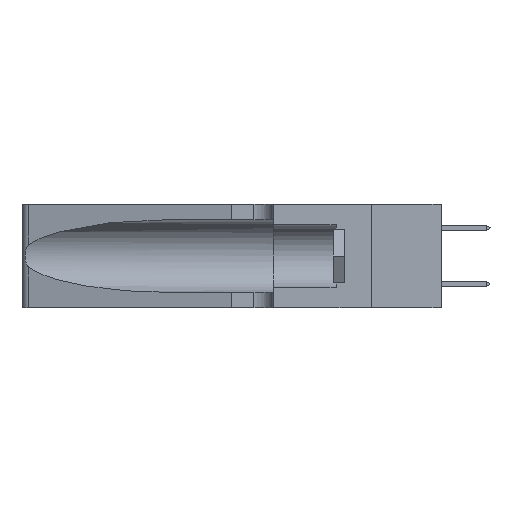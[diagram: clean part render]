
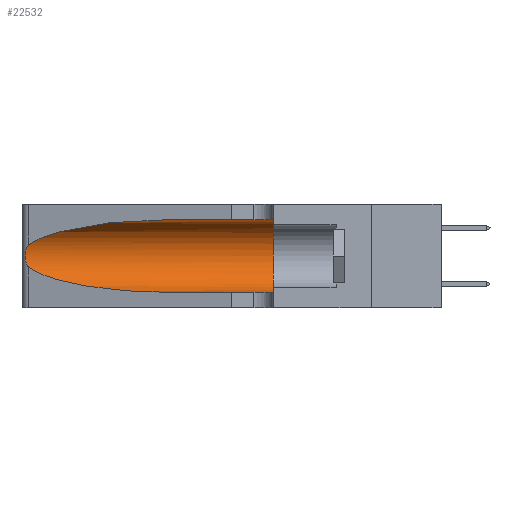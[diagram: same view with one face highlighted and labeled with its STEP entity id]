
A CAD part, left-side view. The second image highlights one B-rep face of the part: STEP entity #22532.
In plain terms, the highlighted cylindrical face has radius 3.308 mm (diameter 6.617 mm), a partial arc.
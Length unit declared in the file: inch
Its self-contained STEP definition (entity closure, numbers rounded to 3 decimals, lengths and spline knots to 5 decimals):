
#297 = CARTESIAN_POINT ( 'NONE',  ( 0.25555, 1.22994, 0.2215 ) ) ;
#299 = VERTEX_POINT ( 'NONE', #20608 ) ;
#329 = VERTEX_POINT ( 'NONE', #12096 ) ;
#825 = CARTESIAN_POINT ( 'NONE',  ( 0.1305, 0.72297, 0.05475 ) ) ;
#1080 = EDGE_CURVE ( 'NONE', #34458, #299, #30667, .T. ) ;
#1246 = LINE ( 'NONE', #26281, #29899 ) ;
#1765 = DIRECTION ( 'NONE',  ( 0., -1., 0. ) ) ;
#2811 = CARTESIAN_POINT ( 'NONE',  ( 0.1305, 0.35, 0.185 ) ) ;
#3085 = CARTESIAN_POINT ( 'NONE',  ( 0.25787, 1.23484, 0.2124 ) ) ;
#3352 = VERTEX_POINT ( 'NONE', #10244 ) ;
#4027 = CYLINDRICAL_SURFACE ( 'NONE', #6193, 0.13025 ) ;
#5576 = DIRECTION ( 'NONE',  ( 0., 0., 1. ) ) ;
#5841 = CARTESIAN_POINT ( 'NONE',  ( 0.26018, 1.23835, 0.19895 ) ) ;
#6193 = AXIS2_PLACEMENT_3D ( 'NONE', #21155, #1765, #29181 ) ;
#7646 = DIRECTION ( 'NONE',  ( 0., -1., 0. ) ) ;
#7833 = AXIS2_PLACEMENT_3D ( 'NONE', #2811, #22202, #5576 ) ;
#8213 = ORIENTED_EDGE ( 'NONE', *, *, #17976, .T. ) ;
#8589 = CARTESIAN_POINT ( 'NONE',  ( 0.26075, 1.23896, 0.178 ) ) ;
#9056 = ORIENTED_EDGE ( 'NONE', *, *, #18629, .T. ) ;
#9939 = CARTESIAN_POINT ( 'NONE',  ( 0.25487, 1.22718, 0.22369 ) ) ;
#10244 = CARTESIAN_POINT ( 'NONE',  ( 0.1305, 0.35, 0.31525 ) ) ;
#11088 = ORIENTED_EDGE ( 'NONE', *, *, #26607, .F. ) ;
#11349 = CARTESIAN_POINT ( 'NONE',  ( 0.25856, 1.23593, 0.16098 ) ) ;
#12096 = CARTESIAN_POINT ( 'NONE',  ( 0.1305, 0.72297, 0.05475 ) ) ;
#12185 = FACE_OUTER_BOUND ( 'NONE', #28134, .T. ) ;
#12963 = ORIENTED_EDGE ( 'NONE', *, *, #1080, .T. ) ;
#14169 = CARTESIAN_POINT ( 'NONE',  ( 0.25639, 1.23186, 0.15144 ) ) ;
#15029 =( BOUNDED_CURVE ( )  B_SPLINE_CURVE ( 3, ( #25590, #31284, #17411, #825 ),
 .UNSPECIFIED., .F., .T. ) 
 B_SPLINE_CURVE_WITH_KNOTS ( ( 4, 4 ),
 ( 3.44316, 4.71239 ),
 .UNSPECIFIED. ) 
 CURVE ( )  GEOMETRIC_REPRESENTATION_ITEM ( )  RATIONAL_B_SPLINE_CURVE ( ( 1., 0.87, 0.87, 1. ) ) 
 REPRESENTATION_ITEM ( '' )  );
#15434 = CARTESIAN_POINT ( 'NONE',  ( 0.1305, 0.72297, 0.31525 ) ) ;
#16083 = EDGE_CURVE ( 'NONE', #19854, #3352, #24612, .T. ) ;
#16888 = CARTESIAN_POINT ( 'NONE',  ( 0.25487, 1.22718, 0.22369 ) ) ;
#17006 = CARTESIAN_POINT ( 'NONE',  ( 0.25487, 1.22718, 0.14631 ) ) ;
#17411 = CARTESIAN_POINT ( 'NONE',  ( 0.18966, 0.96281, 0.05475 ) ) ;
#17976 = EDGE_CURVE ( 'NONE', #299, #329, #15029, .T. ) ;
#18524 = ORIENTED_EDGE ( 'NONE', *, *, #16083, .F. ) ;
#18629 = EDGE_CURVE ( 'NONE', #329, #26020, #1246, .T. ) ;
#19659 = CARTESIAN_POINT ( 'NONE',  ( 0.25639, 1.23184, 0.21858 ) ) ;
#19694 = CARTESIAN_POINT ( 'NONE',  ( 0.1305, 0.72297, 0.31525 ) ) ;
#19854 = VERTEX_POINT ( 'NONE', #19694 ) ;
#20608 = CARTESIAN_POINT ( 'NONE',  ( 0.25487, 1.22718, 0.14631 ) ) ;
#21155 = CARTESIAN_POINT ( 'NONE',  ( 0.1305, 1.61858, 0.185 ) ) ;
#22202 = DIRECTION ( 'NONE',  ( 0., 1., 0. ) ) ;
#22483 = CARTESIAN_POINT ( 'NONE',  ( 0.25854, 1.2359, 0.20912 ) ) ;
#22532 = ADVANCED_FACE ( 'NONE', ( #12185 ), #4027, .F. ) ;
#23453 = ORIENTED_EDGE ( 'NONE', *, *, #35080, .T. ) ;
#23739 = VECTOR ( 'NONE', #7646, 39.37008 ) ;
#24612 = LINE ( 'NONE', #27152, #23739 ) ;
#24699 = CARTESIAN_POINT ( 'NONE',  ( 0.25487, 1.22718, 0.22369 ) ) ;
#24942 = CIRCLE ( 'NONE', #7833, 0.13025 ) ;
#25282 = CARTESIAN_POINT ( 'NONE',  ( 0.26075, 1.23896, 0.19203 ) ) ;
#25590 = CARTESIAN_POINT ( 'NONE',  ( 0.25487, 1.22718, 0.14631 ) ) ;
#26020 = VERTEX_POINT ( 'NONE', #30259 ) ;
#26281 = CARTESIAN_POINT ( 'NONE',  ( 0.1305, 1.61858, 0.05475 ) ) ;
#26607 = EDGE_CURVE ( 'NONE', #3352, #26020, #24942, .T. ) ;
#26684 = CARTESIAN_POINT ( 'NONE',  ( 0.2373, 1.15595, 0.28018 ) ) ;
#27152 = CARTESIAN_POINT ( 'NONE',  ( 0.1305, 1.61858, 0.31525 ) ) ;
#28074 = CARTESIAN_POINT ( 'NONE',  ( 0.26017, 1.23833, 0.17102 ) ) ;
#28134 = EDGE_LOOP ( 'NONE', ( #23453, #12963, #8213, #9056, #11088, #18524 ) ) ;
#29045 = DIRECTION ( 'NONE',  ( 0., -1., 0. ) ) ;
#29181 = DIRECTION ( 'NONE',  ( 0., 0., -1. ) ) ;
#29899 = VECTOR ( 'NONE', #29045, 39.37008 ) ;
#30259 = CARTESIAN_POINT ( 'NONE',  ( 0.1305, 0.35, 0.05475 ) ) ;
#30667 = B_SPLINE_CURVE_WITH_KNOTS ( 'NONE', 3,
 ( #16888, #297, #19659, #3085, #22483, #5841, #25282, #8589, #28074, #11349, #30863, #14169, #33644, #17006 ),
 .UNSPECIFIED., .F., .F.,
 ( 4, 2, 2, 2, 2, 2, 4 ),
 ( 0., 0.00027, 0.00053, 0.00107, 0.0016, 0.00187, 0.00214 ),
 .UNSPECIFIED. ) ;
#30863 = CARTESIAN_POINT ( 'NONE',  ( 0.25789, 1.23486, 0.15765 ) ) ;
#31284 = CARTESIAN_POINT ( 'NONE',  ( 0.2373, 1.15595, 0.08982 ) ) ;
#32106 = CARTESIAN_POINT ( 'NONE',  ( 0.18966, 0.96281, 0.31525 ) ) ;
#33644 = CARTESIAN_POINT ( 'NONE',  ( 0.25555, 1.22993, 0.14849 ) ) ;
#34458 = VERTEX_POINT ( 'NONE', #24699 ) ;
#35080 = EDGE_CURVE ( 'NONE', #19854, #34458, #35533, .T. ) ;
#35533 =( BOUNDED_CURVE ( )  B_SPLINE_CURVE ( 3, ( #15434, #32106, #26684, #9939 ),
 .UNSPECIFIED., .F., .F. ) 
 B_SPLINE_CURVE_WITH_KNOTS ( ( 4, 4 ),
 ( 1.5708, 2.84003 ),
 .UNSPECIFIED. ) 
 CURVE ( )  GEOMETRIC_REPRESENTATION_ITEM ( )  RATIONAL_B_SPLINE_CURVE ( ( 1., 0.87, 0.87, 1. ) ) 
 REPRESENTATION_ITEM ( '' )  );
